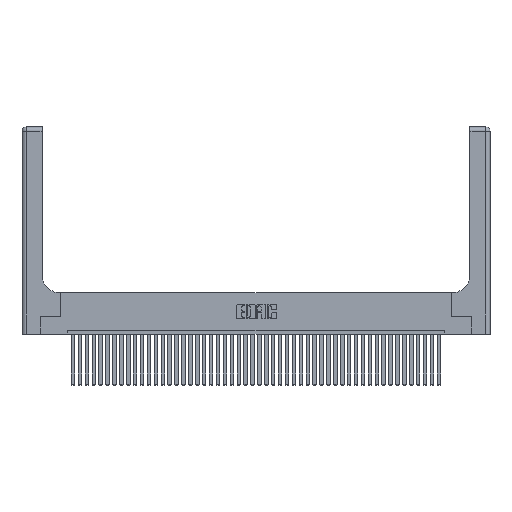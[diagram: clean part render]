
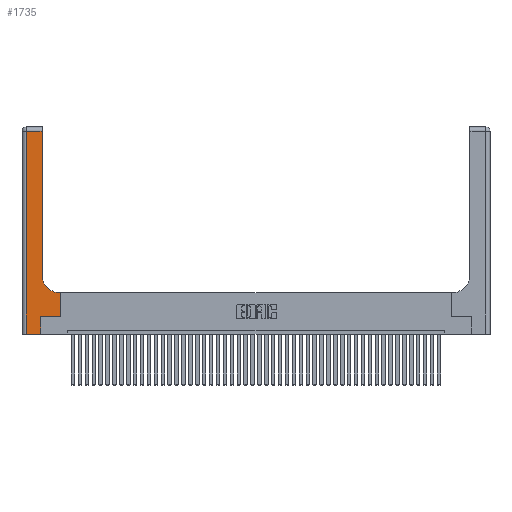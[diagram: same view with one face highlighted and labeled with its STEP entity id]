
A CAD part, top view. The second image highlights one B-rep face of the part: STEP entity #1735.
In plain terms, the highlighted planar face has unit normal (0, 0, 1).
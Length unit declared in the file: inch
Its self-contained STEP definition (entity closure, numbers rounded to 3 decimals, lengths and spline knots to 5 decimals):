
#215 = DIRECTION ( 'NONE',  ( 0., 1., 0. ) ) ;
#404 = ORIENTED_EDGE ( 'NONE', *, *, #29398, .T. ) ;
#664 = VERTEX_POINT ( 'NONE', #21896 ) ;
#1158 = CARTESIAN_POINT ( 'NONE',  ( 0.269, 0., 0.37 ) ) ;
#1735 = ADVANCED_FACE ( 'NONE', ( #17901 ), #36391, .F. ) ;
#3263 = ORIENTED_EDGE ( 'NONE', *, *, #29843, .T. ) ;
#3342 = DIRECTION ( 'NONE',  ( -1., 0., 0. ) ) ;
#3494 = LINE ( 'NONE', #33938, #33280 ) ;
#4300 = ORIENTED_EDGE ( 'NONE', *, *, #15563, .T. ) ;
#5758 = CARTESIAN_POINT ( 'NONE',  ( 0., 2.94, 0.37 ) ) ;
#5789 = DIRECTION ( 'NONE',  ( 0., 0., -1. ) ) ;
#5901 = VECTOR ( 'NONE', #3342, 39.37008 ) ;
#6672 = CARTESIAN_POINT ( 'NONE',  ( 0.2915, 3., 0.37 ) ) ;
#8035 = EDGE_CURVE ( 'NONE', #28851, #10750, #44015, .T. ) ;
#8137 = EDGE_CURVE ( 'NONE', #13866, #16041, #34901, .T. ) ;
#8266 = CARTESIAN_POINT ( 'NONE',  ( 0., 0., 0.37 ) ) ;
#8373 = EDGE_CURVE ( 'NONE', #23962, #33234, #29073, .T. ) ;
#8985 = EDGE_CURVE ( 'NONE', #14015, #664, #3494, .T. ) ;
#9001 = CARTESIAN_POINT ( 'NONE',  ( 0.2915, 2.94, 0.37 ) ) ;
#9649 = ORIENTED_EDGE ( 'NONE', *, *, #8035, .T. ) ;
#10750 = VERTEX_POINT ( 'NONE', #26420 ) ;
#11236 = DIRECTION ( 'NONE',  ( 0., -1., 0. ) ) ;
#11435 = CARTESIAN_POINT ( 'NONE',  ( 0.2915, 0.85, 0.37 ) ) ;
#11508 = DIRECTION ( 'NONE',  ( 1., 0., 0. ) ) ;
#12836 = EDGE_CURVE ( 'NONE', #33234, #28851, #23977, .T. ) ;
#13162 = VECTOR ( 'NONE', #22094, 39.37008 ) ;
#13866 = VERTEX_POINT ( 'NONE', #1158 ) ;
#14015 = VERTEX_POINT ( 'NONE', #35269 ) ;
#14347 = CARTESIAN_POINT ( 'NONE',  ( 0.06, 3., 0.37 ) ) ;
#14537 = EDGE_LOOP ( 'NONE', ( #43388, #33186, #9649, #4300, #33976, #33414, #3263, #30085, #404 ) ) ;
#15199 = CARTESIAN_POINT ( 'NONE',  ( 0.5585, 0.25, 0.37 ) ) ;
#15207 = CIRCLE ( 'NONE', #44033, 0.25 ) ;
#15563 = EDGE_CURVE ( 'NONE', #10750, #13866, #32663, .T. ) ;
#16041 = VERTEX_POINT ( 'NONE', #23145 ) ;
#16693 = EDGE_CURVE ( 'NONE', #16041, #38515, #29144, .T. ) ;
#16954 = LINE ( 'NONE', #18660, #42977 ) ;
#17333 = DIRECTION ( 'NONE',  ( 0., 0., -1. ) ) ;
#17384 = VECTOR ( 'NONE', #11236, 39.37008 ) ;
#17792 = CARTESIAN_POINT ( 'NONE',  ( 0.269, 0.25, 0.37 ) ) ;
#17901 = FACE_OUTER_BOUND ( 'NONE', #14537, .T. ) ;
#18660 = CARTESIAN_POINT ( 'NONE',  ( 0.5585, 0.25, 0.37 ) ) ;
#18798 = CARTESIAN_POINT ( 'NONE',  ( 0.269, 0., 0.37 ) ) ;
#19418 = CARTESIAN_POINT ( 'NONE',  ( 0., 3., 0.37 ) ) ;
#20449 = DIRECTION ( 'NONE',  ( 0., 1., 0. ) ) ;
#21225 = DIRECTION ( 'NONE',  ( 1., 0., 0. ) ) ;
#21896 = CARTESIAN_POINT ( 'NONE',  ( 0.5415, 0.6, 0.37 ) ) ;
#22094 = DIRECTION ( 'NONE',  ( 0., 1., 0. ) ) ;
#23145 = CARTESIAN_POINT ( 'NONE',  ( 0.269, 0.25, 0.37 ) ) ;
#23705 = VECTOR ( 'NONE', #30397, 39.37008 ) ;
#23962 = VERTEX_POINT ( 'NONE', #11435 ) ;
#23977 = LINE ( 'NONE', #5758, #5901 ) ;
#26420 = CARTESIAN_POINT ( 'NONE',  ( 0.06, 0., 0.37 ) ) ;
#28851 = VERTEX_POINT ( 'NONE', #40708 ) ;
#29073 = LINE ( 'NONE', #6672, #30671 ) ;
#29144 = LINE ( 'NONE', #17792, #41898 ) ;
#29398 = EDGE_CURVE ( 'NONE', #664, #23962, #15207, .T. ) ;
#29843 = EDGE_CURVE ( 'NONE', #38515, #14015, #16954, .T. ) ;
#30085 = ORIENTED_EDGE ( 'NONE', *, *, #8985, .T. ) ;
#30397 = DIRECTION ( 'NONE',  ( 1., 0., 0. ) ) ;
#30671 = VECTOR ( 'NONE', #215, 39.37008 ) ;
#32663 = LINE ( 'NONE', #8266, #23705 ) ;
#33186 = ORIENTED_EDGE ( 'NONE', *, *, #12836, .T. ) ;
#33234 = VERTEX_POINT ( 'NONE', #9001 ) ;
#33280 = VECTOR ( 'NONE', #43879, 39.37008 ) ;
#33414 = ORIENTED_EDGE ( 'NONE', *, *, #16693, .T. ) ;
#33938 = CARTESIAN_POINT ( 'NONE',  ( 0.2915, 0.6, 0.37 ) ) ;
#33976 = ORIENTED_EDGE ( 'NONE', *, *, #8137, .T. ) ;
#34901 = LINE ( 'NONE', #18798, #13162 ) ;
#35269 = CARTESIAN_POINT ( 'NONE',  ( 0.5585, 0.6, 0.37 ) ) ;
#36391 = PLANE ( 'NONE',  #36769 ) ;
#36769 = AXIS2_PLACEMENT_3D ( 'NONE', #19418, #5789, #39936 ) ;
#38515 = VERTEX_POINT ( 'NONE', #15199 ) ;
#39936 = DIRECTION ( 'NONE',  ( -1., 0., 0. ) ) ;
#40224 = CARTESIAN_POINT ( 'NONE',  ( 0.5415, 0.85, 0.37 ) ) ;
#40708 = CARTESIAN_POINT ( 'NONE',  ( 0.06, 2.94, 0.37 ) ) ;
#41898 = VECTOR ( 'NONE', #21225, 39.37008 ) ;
#42977 = VECTOR ( 'NONE', #20449, 39.37008 ) ;
#43388 = ORIENTED_EDGE ( 'NONE', *, *, #8373, .T. ) ;
#43879 = DIRECTION ( 'NONE',  ( -1., 0., 0. ) ) ;
#44015 = LINE ( 'NONE', #14347, #17384 ) ;
#44033 = AXIS2_PLACEMENT_3D ( 'NONE', #40224, #17333, #11508 ) ;
